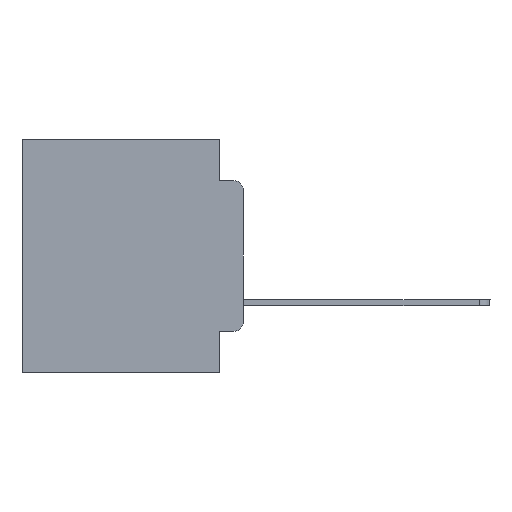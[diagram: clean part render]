
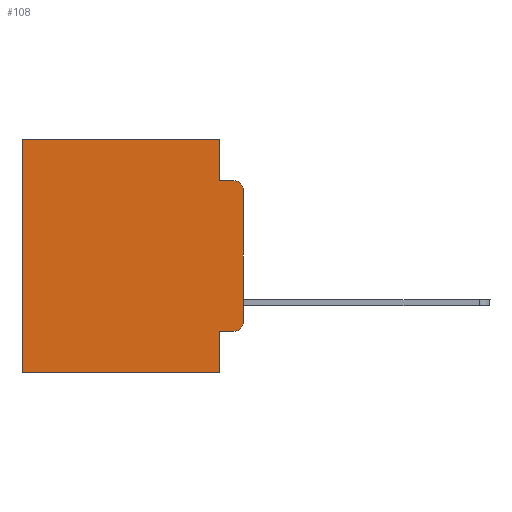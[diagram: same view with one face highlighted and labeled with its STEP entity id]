
A CAD part, left-side view. The second image highlights one B-rep face of the part: STEP entity #108.
In plain terms, the highlighted planar face has unit normal (-1, 0, 0).
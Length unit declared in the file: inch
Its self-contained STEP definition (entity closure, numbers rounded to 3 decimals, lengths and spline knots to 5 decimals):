
#108 = ADVANCED_FACE ( 'NONE', ( #18606 ), #15190, .F. ) ;
#499 = VERTEX_POINT ( 'NONE', #2224 ) ;
#548 = EDGE_CURVE ( 'NONE', #499, #10918, #22945, .T. ) ;
#652 = VERTEX_POINT ( 'NONE', #18170 ) ;
#675 = ORIENTED_EDGE ( 'NONE', *, *, #20298, .T. ) ;
#890 = DIRECTION ( 'NONE',  ( 0., 0., -1. ) ) ;
#974 = DIRECTION ( 'NONE',  ( 0., 0., -1. ) ) ;
#982 = LINE ( 'NONE', #10796, #2322 ) ;
#1492 = EDGE_CURVE ( 'NONE', #6976, #14644, #19535, .T. ) ;
#1580 = EDGE_CURVE ( 'NONE', #4424, #13977, #12500, .T. ) ;
#1655 = VERTEX_POINT ( 'NONE', #25695 ) ;
#2224 = CARTESIAN_POINT ( 'NONE',  ( 0.298, 0., -0.1085 ) ) ;
#2322 = VECTOR ( 'NONE', #20079, 39.37008 ) ;
#2421 = CARTESIAN_POINT ( 'NONE',  ( 0.298, 0.02, -0.4115 ) ) ;
#2518 = VECTOR ( 'NONE', #890, 39.37008 ) ;
#3114 = CARTESIAN_POINT ( 'NONE',  ( 0.298, 0.051, -0.0885 ) ) ;
#3506 = ORIENTED_EDGE ( 'NONE', *, *, #27102, .T. ) ;
#3853 = LINE ( 'NONE', #26251, #2518 ) ;
#4195 = ORIENTED_EDGE ( 'NONE', *, *, #17301, .T. ) ;
#4424 = VERTEX_POINT ( 'NONE', #18981 ) ;
#4790 = ORIENTED_EDGE ( 'NONE', *, *, #548, .F. ) ;
#5018 = CARTESIAN_POINT ( 'NONE',  ( 0.298, 0.02, -0.0885 ) ) ;
#6694 = DIRECTION ( 'NONE',  ( 1., 0., 0. ) ) ;
#6976 = VERTEX_POINT ( 'NONE', #22045 ) ;
#7063 = DIRECTION ( 'NONE',  ( 0., 0., -1. ) ) ;
#7586 = CIRCLE ( 'NONE', #14365, 0.02 ) ;
#7709 = CARTESIAN_POINT ( 'NONE',  ( 0.298, 0.473, 0. ) ) ;
#8772 = DIRECTION ( 'NONE',  ( 0., 0., -1. ) ) ;
#8865 = VECTOR ( 'NONE', #15044, 39.37008 ) ;
#9015 = CARTESIAN_POINT ( 'NONE',  ( 0.298, 0., 0. ) ) ;
#9387 = ORIENTED_EDGE ( 'NONE', *, *, #15302, .F. ) ;
#9522 = CARTESIAN_POINT ( 'NONE',  ( 0.298, 0.051, 0. ) ) ;
#9756 = LINE ( 'NONE', #24923, #26469 ) ;
#10498 = ORIENTED_EDGE ( 'NONE', *, *, #26948, .F. ) ;
#10796 = CARTESIAN_POINT ( 'NONE',  ( 0.298, 0.051, 0. ) ) ;
#10918 = VERTEX_POINT ( 'NONE', #22266 ) ;
#11253 = DIRECTION ( 'NONE',  ( -1., 0., 0. ) ) ;
#12031 = DIRECTION ( 'NONE',  ( 0., -1., 0. ) ) ;
#12500 = LINE ( 'NONE', #21585, #8865 ) ;
#13209 = DIRECTION ( 'NONE',  ( -1., 0., 0. ) ) ;
#13319 = ORIENTED_EDGE ( 'NONE', *, *, #1492, .T. ) ;
#13508 = LINE ( 'NONE', #3114, #25587 ) ;
#13977 = VERTEX_POINT ( 'NONE', #25678 ) ;
#14365 = AXIS2_PLACEMENT_3D ( 'NONE', #17424, #13209, #8772 ) ;
#14560 = LINE ( 'NONE', #9522, #19542 ) ;
#14644 = VERTEX_POINT ( 'NONE', #2421 ) ;
#15044 = DIRECTION ( 'NONE',  ( 0., 1., 0. ) ) ;
#15190 = PLANE ( 'NONE',  #22029 ) ;
#15302 = EDGE_CURVE ( 'NONE', #1655, #652, #982, .T. ) ;
#15673 = VERTEX_POINT ( 'NONE', #7709 ) ;
#17301 = EDGE_CURVE ( 'NONE', #499, #24481, #7586, .T. ) ;
#17410 = DIRECTION ( 'NONE',  ( 0., 0., -1. ) ) ;
#17424 = CARTESIAN_POINT ( 'NONE',  ( 0.298, 0.02, -0.1085 ) ) ;
#18170 = CARTESIAN_POINT ( 'NONE',  ( 0.298, 0.051, -0.0885 ) ) ;
#18178 = VECTOR ( 'NONE', #12031, 39.37008 ) ;
#18380 = DIRECTION ( 'NONE',  ( 0., 1., 0. ) ) ;
#18396 = EDGE_CURVE ( 'NONE', #652, #24481, #13508, .T. ) ;
#18476 = DIRECTION ( 'NONE',  ( 0., 0., -1. ) ) ;
#18606 = FACE_OUTER_BOUND ( 'NONE', #21658, .T. ) ;
#18653 = CARTESIAN_POINT ( 'NONE',  ( 0.298, 0., 0. ) ) ;
#18981 = CARTESIAN_POINT ( 'NONE',  ( 0.298, 0.051, -0.5 ) ) ;
#19535 = LINE ( 'NONE', #24836, #18178 ) ;
#19542 = VECTOR ( 'NONE', #974, 39.37008 ) ;
#20079 = DIRECTION ( 'NONE',  ( 0., 0., -1. ) ) ;
#20298 = EDGE_CURVE ( 'NONE', #1655, #15673, #9756, .T. ) ;
#20380 = ORIENTED_EDGE ( 'NONE', *, *, #1580, .F. ) ;
#20658 = AXIS2_PLACEMENT_3D ( 'NONE', #21736, #11253, #7063 ) ;
#20677 = EDGE_CURVE ( 'NONE', #14644, #10918, #26446, .T. ) ;
#21585 = CARTESIAN_POINT ( 'NONE',  ( 0.298, 0., -0.5 ) ) ;
#21658 = EDGE_LOOP ( 'NONE', ( #4790, #4195, #24141, #9387, #675, #3506, #20380, #10498, #13319, #23686 ) ) ;
#21736 = CARTESIAN_POINT ( 'NONE',  ( 0.298, 0.02, -0.3915 ) ) ;
#22029 = AXIS2_PLACEMENT_3D ( 'NONE', #9015, #6694, #17410 ) ;
#22045 = CARTESIAN_POINT ( 'NONE',  ( 0.298, 0.051, -0.4115 ) ) ;
#22266 = CARTESIAN_POINT ( 'NONE',  ( 0.298, 0., -0.3915 ) ) ;
#22945 = LINE ( 'NONE', #18653, #23277 ) ;
#23277 = VECTOR ( 'NONE', #18476, 39.37008 ) ;
#23686 = ORIENTED_EDGE ( 'NONE', *, *, #20677, .T. ) ;
#24141 = ORIENTED_EDGE ( 'NONE', *, *, #18396, .F. ) ;
#24481 = VERTEX_POINT ( 'NONE', #5018 ) ;
#24836 = CARTESIAN_POINT ( 'NONE',  ( 0.298, 0.051, -0.4115 ) ) ;
#24923 = CARTESIAN_POINT ( 'NONE',  ( 0.298, 0., 0. ) ) ;
#25587 = VECTOR ( 'NONE', #26346, 39.37008 ) ;
#25678 = CARTESIAN_POINT ( 'NONE',  ( 0.298, 0.473, -0.5 ) ) ;
#25695 = CARTESIAN_POINT ( 'NONE',  ( 0.298, 0.051, 0. ) ) ;
#26251 = CARTESIAN_POINT ( 'NONE',  ( 0.298, 0.473, 0. ) ) ;
#26346 = DIRECTION ( 'NONE',  ( 0., -1., 0. ) ) ;
#26446 = CIRCLE ( 'NONE', #20658, 0.02 ) ;
#26469 = VECTOR ( 'NONE', #18380, 39.37008 ) ;
#26948 = EDGE_CURVE ( 'NONE', #6976, #4424, #14560, .T. ) ;
#27102 = EDGE_CURVE ( 'NONE', #15673, #13977, #3853, .T. ) ;
